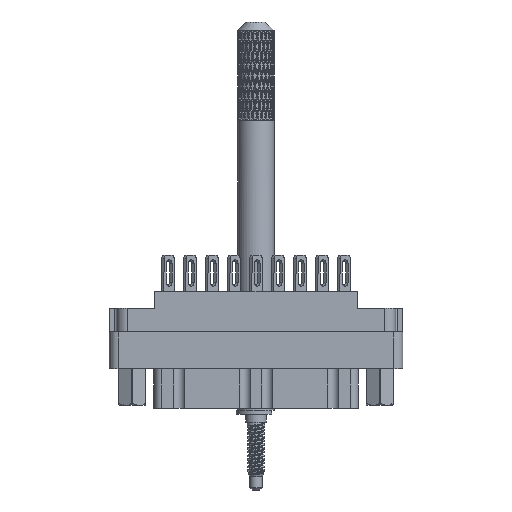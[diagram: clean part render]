
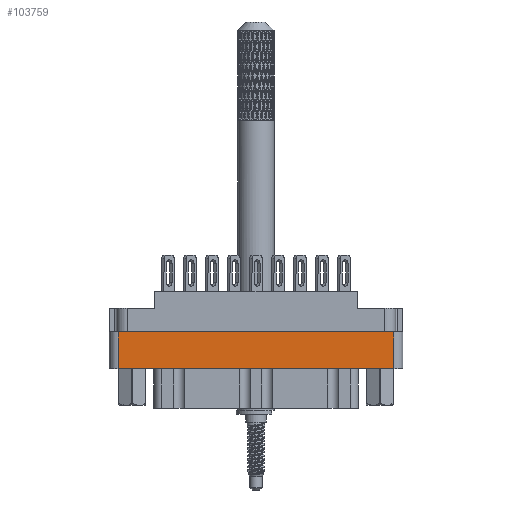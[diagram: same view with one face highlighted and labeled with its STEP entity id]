
A CAD part, front view. The second image highlights one B-rep face of the part: STEP entity #103759.
In plain terms, the highlighted planar face has unit normal (0, -1, 0).
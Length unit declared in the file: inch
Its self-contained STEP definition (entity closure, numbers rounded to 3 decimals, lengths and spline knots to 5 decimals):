
#316 = VERTEX_POINT ( 'NONE', #59968 ) ;
#1097 = LINE ( 'NONE', #29057, #23839 ) ;
#2327 = VECTOR ( 'NONE', #94290, 39.37008 ) ;
#3331 = VERTEX_POINT ( 'NONE', #91747 ) ;
#9528 = ORIENTED_EDGE ( 'NONE', *, *, #29483, .T. ) ;
#10888 = VERTEX_POINT ( 'NONE', #54395 ) ;
#17393 = DIRECTION ( 'NONE',  ( 0., -1., 0. ) ) ;
#18514 = LINE ( 'NONE', #102713, #2327 ) ;
#23839 = VECTOR ( 'NONE', #70655, 39.37008 ) ;
#29057 = CARTESIAN_POINT ( 'NONE',  ( 0.938, -0.438, -0.529 ) ) ;
#29483 = EDGE_CURVE ( 'NONE', #39995, #3331, #18514, .T. ) ;
#30746 = VECTOR ( 'NONE', #44777, 39.37008 ) ;
#39995 = VERTEX_POINT ( 'NONE', #92666 ) ;
#42077 = CARTESIAN_POINT ( 'NONE',  ( -0.938, -0.438, -0.798 ) ) ;
#44777 = DIRECTION ( 'NONE',  ( 0., 0., 1. ) ) ;
#51081 = DIRECTION ( 'NONE',  ( 0., 0., -1. ) ) ;
#54395 = CARTESIAN_POINT ( 'NONE',  ( -0.938, -0.438, -0.529 ) ) ;
#58162 = AXIS2_PLACEMENT_3D ( 'NONE', #42077, #17393, #51081 ) ;
#58945 = FACE_OUTER_BOUND ( 'NONE', #66466, .T. ) ;
#59968 = CARTESIAN_POINT ( 'NONE',  ( -0.938, -0.438, -0.277 ) ) ;
#63307 = DIRECTION ( 'NONE',  ( 1., 0., 0. ) ) ;
#63430 = ORIENTED_EDGE ( 'NONE', *, *, #77262, .F. ) ;
#63950 = EDGE_CURVE ( 'NONE', #39995, #10888, #1097, .T. ) ;
#66466 = EDGE_LOOP ( 'NONE', ( #103567, #88649, #9528, #63430 ) ) ;
#70655 = DIRECTION ( 'NONE',  ( -1., 0., 0. ) ) ;
#77262 = EDGE_CURVE ( 'NONE', #316, #3331, #87963, .T. ) ;
#78012 = PLANE ( 'NONE',  #58162 ) ;
#80665 = CARTESIAN_POINT ( 'NONE',  ( -1., -0.438, -0.277 ) ) ;
#87781 = VECTOR ( 'NONE', #63307, 39.37008 ) ;
#87963 = LINE ( 'NONE', #80665, #87781 ) ;
#88649 = ORIENTED_EDGE ( 'NONE', *, *, #63950, .F. ) ;
#91747 = CARTESIAN_POINT ( 'NONE',  ( 0.938, -0.438, -0.277 ) ) ;
#92666 = CARTESIAN_POINT ( 'NONE',  ( 0.938, -0.438, -0.529 ) ) ;
#94290 = DIRECTION ( 'NONE',  ( 0., 0., 1. ) ) ;
#98075 = CARTESIAN_POINT ( 'NONE',  ( -0.938, -0.438, -0.798 ) ) ;
#102713 = CARTESIAN_POINT ( 'NONE',  ( 0.938, -0.438, -0.798 ) ) ;
#103567 = ORIENTED_EDGE ( 'NONE', *, *, #110332, .F. ) ;
#103759 = ADVANCED_FACE ( 'NONE', ( #58945 ), #78012, .T. ) ;
#106506 = LINE ( 'NONE', #98075, #30746 ) ;
#110332 = EDGE_CURVE ( 'NONE', #10888, #316, #106506, .T. ) ;
